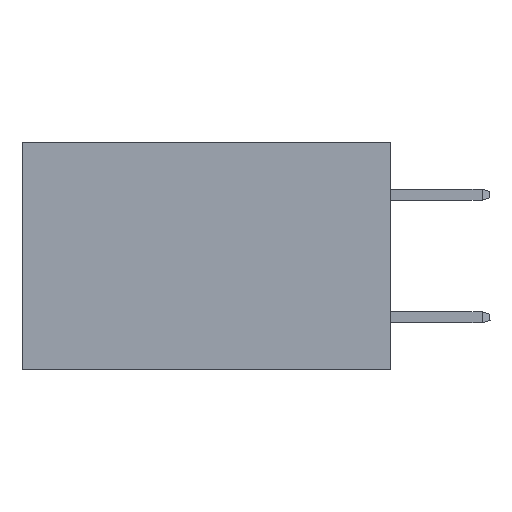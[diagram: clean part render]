
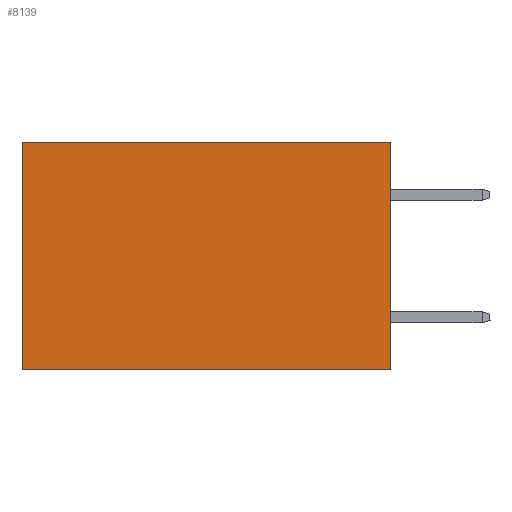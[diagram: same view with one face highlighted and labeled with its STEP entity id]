
A CAD part, left-side view. The second image highlights one B-rep face of the part: STEP entity #8139.
In plain terms, the highlighted planar face has unit normal (-1, 0, 0).
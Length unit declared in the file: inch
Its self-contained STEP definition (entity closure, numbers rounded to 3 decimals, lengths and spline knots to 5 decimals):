
#443 = VECTOR ( 'NONE', #12919, 39.37008 ) ;
#839 = CARTESIAN_POINT ( 'NONE',  ( 0.2875, 0.6, -0.37 ) ) ;
#870 = LINE ( 'NONE', #10313, #443 ) ;
#1285 = VECTOR ( 'NONE', #9943, 39.37008 ) ;
#1327 = CARTESIAN_POINT ( 'NONE',  ( 0.2875, 0., 0. ) ) ;
#1896 = CARTESIAN_POINT ( 'NONE',  ( 0.2875, 0., 0. ) ) ;
#2660 = DIRECTION ( 'NONE',  ( 0., 0., -1. ) ) ;
#2838 = VERTEX_POINT ( 'NONE', #4940 ) ;
#3037 = ORIENTED_EDGE ( 'NONE', *, *, #4292, .T. ) ;
#3341 = FACE_OUTER_BOUND ( 'NONE', #14929, .T. ) ;
#4292 = EDGE_CURVE ( 'NONE', #15670, #11710, #11851, .T. ) ;
#4497 = LINE ( 'NONE', #1896, #1285 ) ;
#4940 = CARTESIAN_POINT ( 'NONE',  ( 0.2875, 0., 0. ) ) ;
#5119 = EDGE_CURVE ( 'NONE', #2838, #7259, #11990, .T. ) ;
#6102 = EDGE_CURVE ( 'NONE', #7259, #11710, #870, .T. ) ;
#6562 = EDGE_CURVE ( 'NONE', #2838, #15670, #4497, .T. ) ;
#6753 = ORIENTED_EDGE ( 'NONE', *, *, #6562, .T. ) ;
#7259 = VERTEX_POINT ( 'NONE', #16713 ) ;
#8108 = VECTOR ( 'NONE', #16842, 39.37008 ) ;
#8139 = ADVANCED_FACE ( 'NONE', ( #3341 ), #17136, .F. ) ;
#8464 = AXIS2_PLACEMENT_3D ( 'NONE', #1327, #10712, #2660 ) ;
#8790 = VECTOR ( 'NONE', #10591, 39.37008 ) ;
#9360 = CARTESIAN_POINT ( 'NONE',  ( 0.2875, 0.6, 0. ) ) ;
#9943 = DIRECTION ( 'NONE',  ( 0., 1., 0. ) ) ;
#10313 = CARTESIAN_POINT ( 'NONE',  ( 0.2875, 0., -0.37 ) ) ;
#10523 = CARTESIAN_POINT ( 'NONE',  ( 0.2875, 0.6, 0. ) ) ;
#10591 = DIRECTION ( 'NONE',  ( 0., 0., -1. ) ) ;
#10712 = DIRECTION ( 'NONE',  ( 1., 0., 0. ) ) ;
#11710 = VERTEX_POINT ( 'NONE', #839 ) ;
#11851 = LINE ( 'NONE', #10523, #8790 ) ;
#11990 = LINE ( 'NONE', #13519, #8108 ) ;
#12919 = DIRECTION ( 'NONE',  ( 0., 1., 0. ) ) ;
#13519 = CARTESIAN_POINT ( 'NONE',  ( 0.2875, 0., 0. ) ) ;
#14929 = EDGE_LOOP ( 'NONE', ( #3037, #16957, #15673, #6753 ) ) ;
#15670 = VERTEX_POINT ( 'NONE', #9360 ) ;
#15673 = ORIENTED_EDGE ( 'NONE', *, *, #5119, .F. ) ;
#16713 = CARTESIAN_POINT ( 'NONE',  ( 0.2875, 0., -0.37 ) ) ;
#16842 = DIRECTION ( 'NONE',  ( 0., 0., -1. ) ) ;
#16957 = ORIENTED_EDGE ( 'NONE', *, *, #6102, .F. ) ;
#17136 = PLANE ( 'NONE',  #8464 ) ;
